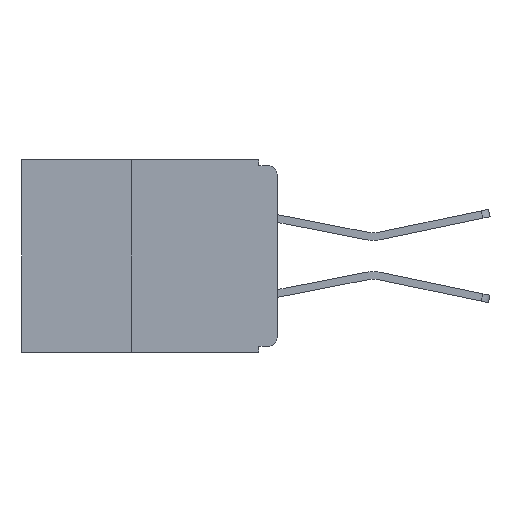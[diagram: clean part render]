
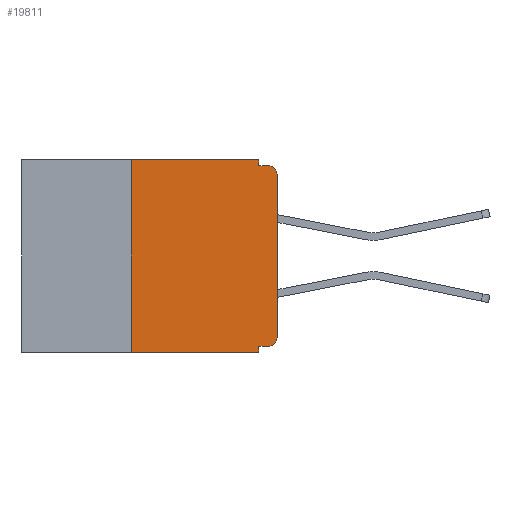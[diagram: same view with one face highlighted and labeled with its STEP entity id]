
A CAD part, left-side view. The second image highlights one B-rep face of the part: STEP entity #19811.
In plain terms, the highlighted planar face has unit normal (-1, 0, 0).
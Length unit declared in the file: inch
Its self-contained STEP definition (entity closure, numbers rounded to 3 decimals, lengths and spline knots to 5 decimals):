
#407 = CARTESIAN_POINT ( 'NONE',  ( 0., 0.25, -0.33 ) ) ;
#675 = EDGE_CURVE ( 'NONE', #10921, #9149, #27049, .T. ) ;
#1078 = DIRECTION ( 'NONE',  ( 0., 0., -1. ) ) ;
#1270 = LINE ( 'NONE', #12907, #18856 ) ;
#1559 = CARTESIAN_POINT ( 'NONE',  ( 0., 0.031, -0.33 ) ) ;
#1772 = CARTESIAN_POINT ( 'NONE',  ( 0., 0.031, -0.01 ) ) ;
#2038 = CARTESIAN_POINT ( 'NONE',  ( 0., 0., -0.32 ) ) ;
#2050 = CARTESIAN_POINT ( 'NONE',  ( 0., 0., -0.01 ) ) ;
#2122 = LINE ( 'NONE', #1559, #12929 ) ;
#2387 = EDGE_CURVE ( 'NONE', #17331, #14271, #2122, .T. ) ;
#2728 = AXIS2_PLACEMENT_3D ( 'NONE', #4536, #20555, #6839 ) ;
#2797 = LINE ( 'NONE', #2038, #14343 ) ;
#2902 = CARTESIAN_POINT ( 'NONE',  ( 0., 0.437, 0. ) ) ;
#3622 = ORIENTED_EDGE ( 'NONE', *, *, #8540, .F. ) ;
#3851 = LINE ( 'NONE', #2050, #16124 ) ;
#4536 = CARTESIAN_POINT ( 'NONE',  ( 0., 0.015, -0.025 ) ) ;
#4710 = ORIENTED_EDGE ( 'NONE', *, *, #16123, .F. ) ;
#5310 = EDGE_CURVE ( 'NONE', #29052, #25777, #14982, .T. ) ;
#5455 = ORIENTED_EDGE ( 'NONE', *, *, #8359, .F. ) ;
#6684 = LINE ( 'NONE', #8048, #16080 ) ;
#6839 = DIRECTION ( 'NONE',  ( 0., 0., -1. ) ) ;
#7007 = EDGE_CURVE ( 'NONE', #17737, #14271, #17713, .T. ) ;
#8048 = CARTESIAN_POINT ( 'NONE',  ( 0., 0.031, 0. ) ) ;
#8359 = EDGE_CURVE ( 'NONE', #10921, #17331, #2797, .T. ) ;
#8540 = EDGE_CURVE ( 'NONE', #17737, #20846, #17550, .T. ) ;
#8606 = CARTESIAN_POINT ( 'NONE',  ( 0., 0., -0.025 ) ) ;
#9149 = VERTEX_POINT ( 'NONE', #14086 ) ;
#9656 = CARTESIAN_POINT ( 'NONE',  ( 0., 0.031, 0. ) ) ;
#9890 = EDGE_CURVE ( 'NONE', #20846, #14518, #27717, .T. ) ;
#10097 = EDGE_CURVE ( 'NONE', #14518, #20599, #6684, .T. ) ;
#10555 = DIRECTION ( 'NONE',  ( 0., 0., 1. ) ) ;
#10921 = VERTEX_POINT ( 'NONE', #20158 ) ;
#11009 = AXIS2_PLACEMENT_3D ( 'NONE', #2902, #28023, #14503 ) ;
#11025 = VECTOR ( 'NONE', #11996, 39.37008 ) ;
#11561 = ORIENTED_EDGE ( 'NONE', *, *, #675, .T. ) ;
#11996 = DIRECTION ( 'NONE',  ( 0., -1., 0. ) ) ;
#12907 = CARTESIAN_POINT ( 'NONE',  ( 0., 0., 0. ) ) ;
#12929 = VECTOR ( 'NONE', #1078, 39.37008 ) ;
#13000 = ORIENTED_EDGE ( 'NONE', *, *, #9890, .F. ) ;
#13374 = ORIENTED_EDGE ( 'NONE', *, *, #2387, .F. ) ;
#13579 = CARTESIAN_POINT ( 'NONE',  ( 0., 0.437, -0.33 ) ) ;
#14086 = CARTESIAN_POINT ( 'NONE',  ( 0., 0., -0.305 ) ) ;
#14218 = DIRECTION ( 'NONE',  ( 0., 0., 1. ) ) ;
#14271 = VERTEX_POINT ( 'NONE', #22449 ) ;
#14343 = VECTOR ( 'NONE', #20374, 39.37008 ) ;
#14503 = DIRECTION ( 'NONE',  ( 0., 0., -1. ) ) ;
#14518 = VERTEX_POINT ( 'NONE', #9656 ) ;
#14982 = CIRCLE ( 'NONE', #2728, 0.015 ) ;
#15857 = DIRECTION ( 'NONE',  ( 0., -1., 0. ) ) ;
#16080 = VECTOR ( 'NONE', #17240, 39.37008 ) ;
#16123 = EDGE_CURVE ( 'NONE', #20599, #25777, #3851, .T. ) ;
#16124 = VECTOR ( 'NONE', #15857, 39.37008 ) ;
#16133 = VECTOR ( 'NONE', #14218, 39.37008 ) ;
#17240 = DIRECTION ( 'NONE',  ( 0., 0., -1. ) ) ;
#17331 = VERTEX_POINT ( 'NONE', #18987 ) ;
#17550 = LINE ( 'NONE', #407, #16133 ) ;
#17713 = LINE ( 'NONE', #13579, #22982 ) ;
#17737 = VERTEX_POINT ( 'NONE', #29383 ) ;
#18615 = CARTESIAN_POINT ( 'NONE',  ( 0., 0.25, 0. ) ) ;
#18856 = VECTOR ( 'NONE', #10555, 39.37008 ) ;
#18987 = CARTESIAN_POINT ( 'NONE',  ( 0., 0.031, -0.32 ) ) ;
#19135 = DIRECTION ( 'NONE',  ( 0., 0., -1. ) ) ;
#19271 = CARTESIAN_POINT ( 'NONE',  ( 0., 0.015, -0.305 ) ) ;
#19295 = DIRECTION ( 'NONE',  ( -1., 0., 0. ) ) ;
#19811 = ADVANCED_FACE ( 'NONE', ( #26831 ), #25776, .F. ) ;
#20149 = AXIS2_PLACEMENT_3D ( 'NONE', #19271, #19295, #19135 ) ;
#20158 = CARTESIAN_POINT ( 'NONE',  ( 0., 0.015, -0.32 ) ) ;
#20374 = DIRECTION ( 'NONE',  ( 0., 1., 0. ) ) ;
#20555 = DIRECTION ( 'NONE',  ( -1., 0., 0. ) ) ;
#20599 = VERTEX_POINT ( 'NONE', #1772 ) ;
#20829 = ORIENTED_EDGE ( 'NONE', *, *, #25192, .T. ) ;
#20846 = VERTEX_POINT ( 'NONE', #18615 ) ;
#22449 = CARTESIAN_POINT ( 'NONE',  ( 0., 0.031, -0.33 ) ) ;
#22940 = ORIENTED_EDGE ( 'NONE', *, *, #10097, .F. ) ;
#22982 = VECTOR ( 'NONE', #24883, 39.37008 ) ;
#23514 = CARTESIAN_POINT ( 'NONE',  ( 0., 0.015, -0.01 ) ) ;
#24883 = DIRECTION ( 'NONE',  ( 0., -1., 0. ) ) ;
#25192 = EDGE_CURVE ( 'NONE', #9149, #29052, #1270, .T. ) ;
#25623 = CARTESIAN_POINT ( 'NONE',  ( 0., 0.437, 0. ) ) ;
#25776 = PLANE ( 'NONE',  #11009 ) ;
#25777 = VERTEX_POINT ( 'NONE', #23514 ) ;
#26831 = FACE_OUTER_BOUND ( 'NONE', #28086, .T. ) ;
#26834 = ORIENTED_EDGE ( 'NONE', *, *, #5310, .T. ) ;
#27049 = CIRCLE ( 'NONE', #20149, 0.015 ) ;
#27717 = LINE ( 'NONE', #25623, #11025 ) ;
#28023 = DIRECTION ( 'NONE',  ( 1., 0., 0. ) ) ;
#28086 = EDGE_LOOP ( 'NONE', ( #20829, #26834, #4710, #22940, #13000, #3622, #29289, #13374, #5455, #11561 ) ) ;
#29052 = VERTEX_POINT ( 'NONE', #8606 ) ;
#29289 = ORIENTED_EDGE ( 'NONE', *, *, #7007, .T. ) ;
#29383 = CARTESIAN_POINT ( 'NONE',  ( 0., 0.25, -0.33 ) ) ;
